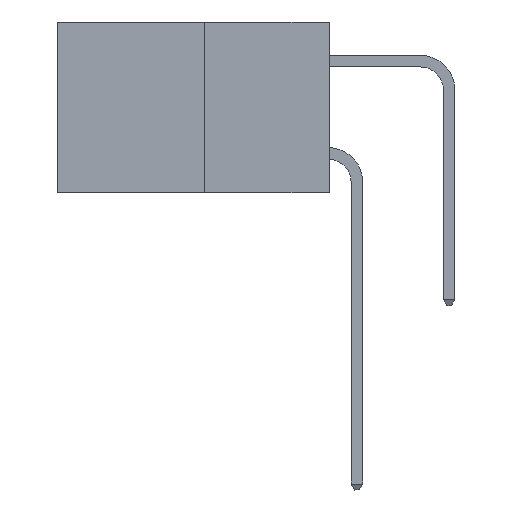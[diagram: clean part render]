
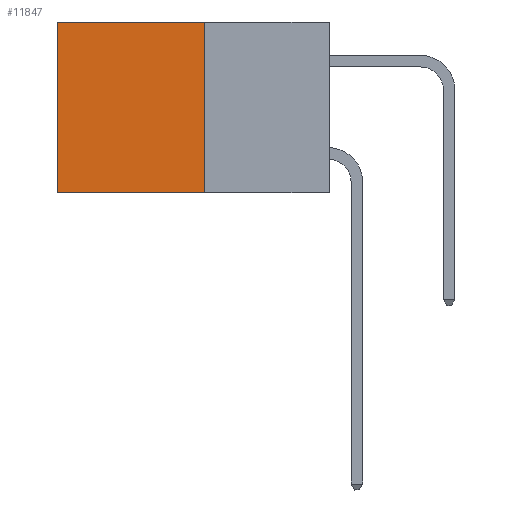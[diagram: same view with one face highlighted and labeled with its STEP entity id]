
A CAD part, left-side view. The second image highlights one B-rep face of the part: STEP entity #11847.
In plain terms, the highlighted planar face has unit normal (-1, 0, 0).
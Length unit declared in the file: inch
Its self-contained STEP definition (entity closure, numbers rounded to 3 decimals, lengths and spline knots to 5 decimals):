
#857 = CARTESIAN_POINT ( 'NONE',  ( 0.277, 0.27, 0. ) ) ;
#1135 = VECTOR ( 'NONE', #4736, 39.37008 ) ;
#1208 = ORIENTED_EDGE ( 'NONE', *, *, #8131, .F. ) ;
#1250 = CARTESIAN_POINT ( 'NONE',  ( 0.277, 0.27, -0.37 ) ) ;
#1737 = VERTEX_POINT ( 'NONE', #4062 ) ;
#2633 = EDGE_CURVE ( 'NONE', #1737, #4077, #3874, .T. ) ;
#2761 = CARTESIAN_POINT ( 'NONE',  ( 0.277, 0.59, 0. ) ) ;
#3111 = ORIENTED_EDGE ( 'NONE', *, *, #10703, .T. ) ;
#3440 = VECTOR ( 'NONE', #6232, 39.37008 ) ;
#3512 = VERTEX_POINT ( 'NONE', #2761 ) ;
#3736 = LINE ( 'NONE', #5289, #3440 ) ;
#3826 = DIRECTION ( 'NONE',  ( 0., 0., -1. ) ) ;
#3874 = LINE ( 'NONE', #5103, #8886 ) ;
#4062 = CARTESIAN_POINT ( 'NONE',  ( 0.277, 0.27, -0.37 ) ) ;
#4077 = VERTEX_POINT ( 'NONE', #7769 ) ;
#4176 = DIRECTION ( 'NONE',  ( 0., 0., -1. ) ) ;
#4565 = EDGE_LOOP ( 'NONE', ( #3111, #10874, #1208, #6539 ) ) ;
#4736 = DIRECTION ( 'NONE',  ( 0., 1., 0. ) ) ;
#5103 = CARTESIAN_POINT ( 'NONE',  ( 0.277, 0.27, -0.37 ) ) ;
#5289 = CARTESIAN_POINT ( 'NONE',  ( 0.277, 0.27, -0.37 ) ) ;
#5780 = DIRECTION ( 'NONE',  ( 0., 1., 0. ) ) ;
#6225 = LINE ( 'NONE', #7527, #1135 ) ;
#6232 = DIRECTION ( 'NONE',  ( 0., 0., -1. ) ) ;
#6515 = AXIS2_PLACEMENT_3D ( 'NONE', #1250, #9794, #4176 ) ;
#6539 = ORIENTED_EDGE ( 'NONE', *, *, #8999, .T. ) ;
#7527 = CARTESIAN_POINT ( 'NONE',  ( 0.277, 0.27, 0. ) ) ;
#7769 = CARTESIAN_POINT ( 'NONE',  ( 0.277, 0.59, -0.37 ) ) ;
#7922 = PLANE ( 'NONE',  #6515 ) ;
#8131 = EDGE_CURVE ( 'NONE', #12225, #1737, #3736, .T. ) ;
#8533 = CARTESIAN_POINT ( 'NONE',  ( 0.277, 0.59, -0.37 ) ) ;
#8886 = VECTOR ( 'NONE', #5780, 39.37008 ) ;
#8999 = EDGE_CURVE ( 'NONE', #12225, #3512, #6225, .T. ) ;
#9794 = DIRECTION ( 'NONE',  ( 1., 0., 0. ) ) ;
#10299 = VECTOR ( 'NONE', #3826, 39.37008 ) ;
#10703 = EDGE_CURVE ( 'NONE', #3512, #4077, #12177, .T. ) ;
#10874 = ORIENTED_EDGE ( 'NONE', *, *, #2633, .F. ) ;
#11847 = ADVANCED_FACE ( 'NONE', ( #12287 ), #7922, .F. ) ;
#12177 = LINE ( 'NONE', #8533, #10299 ) ;
#12225 = VERTEX_POINT ( 'NONE', #857 ) ;
#12287 = FACE_OUTER_BOUND ( 'NONE', #4565, .T. ) ;
